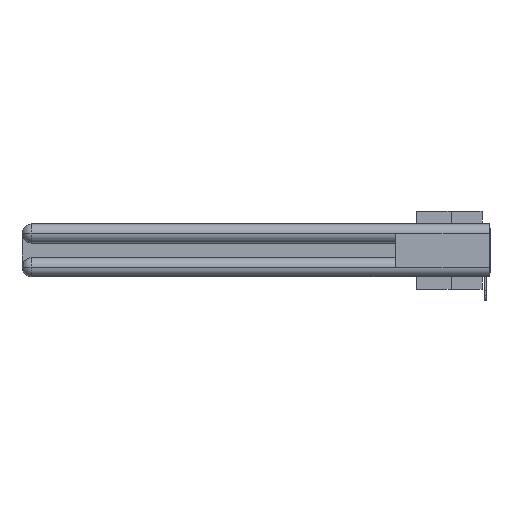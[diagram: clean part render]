
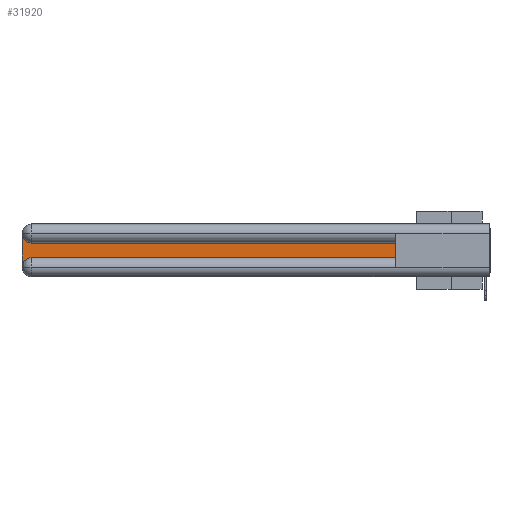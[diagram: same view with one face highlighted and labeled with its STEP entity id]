
A CAD part, left-side view. The second image highlights one B-rep face of the part: STEP entity #31920.
In plain terms, the highlighted planar face has unit normal (-1, 0, 0).
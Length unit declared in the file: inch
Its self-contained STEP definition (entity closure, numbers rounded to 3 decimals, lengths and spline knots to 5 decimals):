
#1491 = VECTOR ( 'NONE', #35033, 39.37008 ) ;
#1586 = VERTEX_POINT ( 'NONE', #5828 ) ;
#2194 = AXIS2_PLACEMENT_3D ( 'NONE', #33703, #9304, #31017 ) ;
#2229 = CARTESIAN_POINT ( 'NONE',  ( 0.075, 0.6, -0.1225 ) ) ;
#2296 = CARTESIAN_POINT ( 'NONE',  ( 0.075, 0.6, -0.1225 ) ) ;
#3522 = DIRECTION ( 'NONE',  ( 0., 0., -1. ) ) ;
#3538 = CARTESIAN_POINT ( 'NONE',  ( 0.075, 3., -0.0625 ) ) ;
#4505 = EDGE_CURVE ( 'NONE', #25591, #1586, #28247, .T. ) ;
#5378 = PLANE ( 'NONE',  #16963 ) ;
#5828 = CARTESIAN_POINT ( 'NONE',  ( 0.075, 3., -0.2775 ) ) ;
#6106 = EDGE_CURVE ( 'NONE', #16673, #23478, #32703, .T. ) ;
#6323 = EDGE_LOOP ( 'NONE', ( #17183, #7729, #13520, #28280, #6934, #10842 ) ) ;
#6367 = CARTESIAN_POINT ( 'NONE',  ( 0.075, 3., -0.2175 ) ) ;
#6934 = ORIENTED_EDGE ( 'NONE', *, *, #6106, .T. ) ;
#7729 = ORIENTED_EDGE ( 'NONE', *, *, #14106, .T. ) ;
#9304 = DIRECTION ( 'NONE',  ( 1., 0., 0. ) ) ;
#10599 = DIRECTION ( 'NONE',  ( 0., 0., 1. ) ) ;
#10842 = ORIENTED_EDGE ( 'NONE', *, *, #34455, .T. ) ;
#13095 = CARTESIAN_POINT ( 'NONE',  ( 0.075, 0.6, -0.2175 ) ) ;
#13162 = DIRECTION ( 'NONE',  ( 0., 0., -1. ) ) ;
#13520 = ORIENTED_EDGE ( 'NONE', *, *, #4505, .T. ) ;
#13788 = LINE ( 'NONE', #2229, #25567 ) ;
#14050 = CARTESIAN_POINT ( 'NONE',  ( 0.075, 2.94, -0.1225 ) ) ;
#14106 = EDGE_CURVE ( 'NONE', #26632, #25591, #14819, .T. ) ;
#14819 = CIRCLE ( 'NONE', #34175, 0.06 ) ;
#15809 = VECTOR ( 'NONE', #3522, 39.37008 ) ;
#15935 = DIRECTION ( 'NONE',  ( 0., 1., 0. ) ) ;
#16673 = VERTEX_POINT ( 'NONE', #19339 ) ;
#16963 = AXIS2_PLACEMENT_3D ( 'NONE', #19065, #34587, #31916 ) ;
#17183 = ORIENTED_EDGE ( 'NONE', *, *, #20742, .T. ) ;
#18421 = LINE ( 'NONE', #13095, #24482 ) ;
#18815 = CARTESIAN_POINT ( 'NONE',  ( 0.075, 0.6, -0.2175 ) ) ;
#19065 = CARTESIAN_POINT ( 'NONE',  ( 0.075, 3., -0.1225 ) ) ;
#19339 = CARTESIAN_POINT ( 'NONE',  ( 0.075, 2.94, -0.2175 ) ) ;
#20508 = CARTESIAN_POINT ( 'NONE',  ( 0.075, 0.6, -0.2175 ) ) ;
#20742 = EDGE_CURVE ( 'NONE', #29547, #26632, #13788, .T. ) ;
#20989 = DIRECTION ( 'NONE',  ( 1., 0., 0. ) ) ;
#21172 = CARTESIAN_POINT ( 'NONE',  ( 0.075, 2.94, -0.0625 ) ) ;
#23478 = VERTEX_POINT ( 'NONE', #20508 ) ;
#24482 = VECTOR ( 'NONE', #10599, 39.37008 ) ;
#25567 = VECTOR ( 'NONE', #15935, 39.37008 ) ;
#25591 = VERTEX_POINT ( 'NONE', #3538 ) ;
#26632 = VERTEX_POINT ( 'NONE', #14050 ) ;
#28247 = LINE ( 'NONE', #6367, #15809 ) ;
#28280 = ORIENTED_EDGE ( 'NONE', *, *, #31861, .T. ) ;
#29405 = FACE_OUTER_BOUND ( 'NONE', #6323, .T. ) ;
#29475 = CIRCLE ( 'NONE', #2194, 0.06 ) ;
#29547 = VERTEX_POINT ( 'NONE', #2296 ) ;
#31017 = DIRECTION ( 'NONE',  ( 0., 0., -1. ) ) ;
#31861 = EDGE_CURVE ( 'NONE', #1586, #16673, #29475, .T. ) ;
#31916 = DIRECTION ( 'NONE',  ( 0., 0., -1. ) ) ;
#31920 = ADVANCED_FACE ( 'NONE', ( #29405 ), #5378, .F. ) ;
#32703 = LINE ( 'NONE', #18815, #1491 ) ;
#33703 = CARTESIAN_POINT ( 'NONE',  ( 0.075, 2.94, -0.2775 ) ) ;
#34175 = AXIS2_PLACEMENT_3D ( 'NONE', #21172, #20989, #13162 ) ;
#34455 = EDGE_CURVE ( 'NONE', #23478, #29547, #18421, .T. ) ;
#34587 = DIRECTION ( 'NONE',  ( 1., 0., 0. ) ) ;
#35033 = DIRECTION ( 'NONE',  ( 0., -1., 0. ) ) ;
